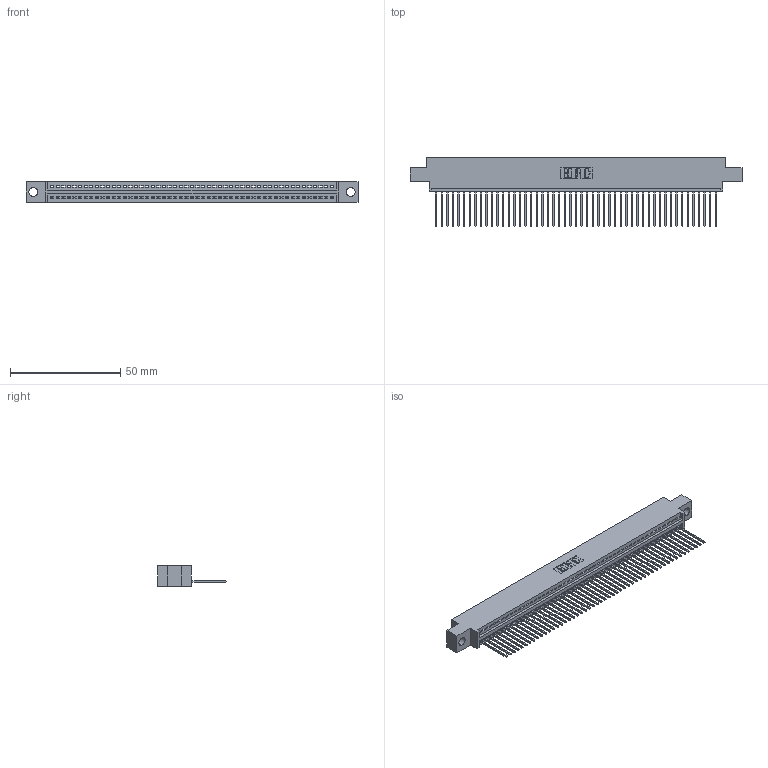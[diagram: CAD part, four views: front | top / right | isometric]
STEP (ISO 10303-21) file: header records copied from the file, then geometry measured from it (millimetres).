
FILE_DESCRIPTION (( 'STEP AP203' ), '1' );
FILE_NAME ('345-051-542-604.STEP', '2021-05-28T15:24:45', ( '' ), ( '' ), 'SwSTEP 2.0', 'SolidWorks 2020', '' );
FILE_SCHEMA (( 'CONFIG_CONTROL_DESIGN' ));
Length unit declared in the file: inch
Products named in the file (3): 345-292-001_345-293-142; 345 Part_0.170 Offset - 0.156 Dia-TI; 345-051-542-604
Assembly tree (52 placements, depth 2):
  345-051-542-604
    345 Part_0.170 Offset - 0.156 Dia-TI
    345-292-001_345-293-142  x51
Bounding box: 150.75 x 31.29 x 9.4 mm (x, y, z)
Volume: 14286.1 mm3; surface area: 19793.9 mm2
Topology: 52 solids, 52 shells, 3102 faces, 9365 edges, 6174 vertices
Faces by surface type: plane 2138, cylinder 964
Entity records: 37741 total; most frequent: CARTESIAN_POINT 6547, ORIENTED_EDGE 6530, DIRECTION 5703, EDGE_CURVE 3265, LINE 2929, VECTOR 2929, VERTEX_POINT 2174, AXIS2_PLACEMENT_3D 1387
